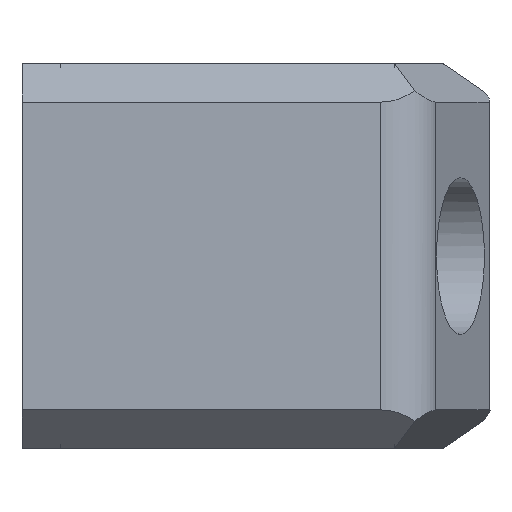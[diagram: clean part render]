
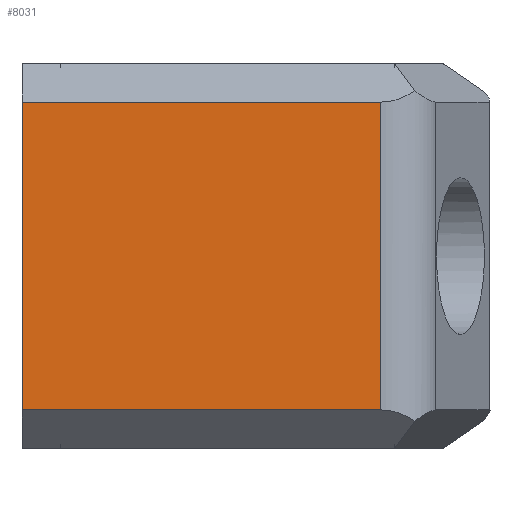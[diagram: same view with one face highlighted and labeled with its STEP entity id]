
A CAD part, left-side view. The second image highlights one B-rep face of the part: STEP entity #8031.
In plain terms, the highlighted planar face has unit normal (-1, 0, 0).
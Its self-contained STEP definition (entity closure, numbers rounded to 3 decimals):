
#233=PLANE('',#8473);
#665=FACE_OUTER_BOUND('',#1100,.T.);
#1100=EDGE_LOOP('',(#5845,#5846,#5847,#5848));
#1524=LINE('',#10746,#2566);
#1534=LINE('',#12873,#2576);
#1538=LINE('',#12881,#2580);
#1539=LINE('',#12882,#2581);
#2566=VECTOR('',#8887,10.);
#2576=VECTOR('',#8939,10.);
#2580=VECTOR('',#8945,10.);
#2581=VECTOR('',#8946,10.);
#3623=VERTEX_POINT('',#10743);
#3624=VERTEX_POINT('',#10745);
#3702=VERTEX_POINT('',#12872);
#3705=VERTEX_POINT('',#12880);
#4420=EDGE_CURVE('',#3623,#3624,#1524,.T.);
#4535=EDGE_CURVE('',#3624,#3702,#1534,.T.);
#4539=EDGE_CURVE('',#3705,#3623,#1538,.T.);
#4540=EDGE_CURVE('',#3702,#3705,#1539,.T.);
#5845=ORIENTED_EDGE('',*,*,#4420,.F.);
#5846=ORIENTED_EDGE('',*,*,#4539,.F.);
#5847=ORIENTED_EDGE('',*,*,#4540,.F.);
#5848=ORIENTED_EDGE('',*,*,#4535,.F.);
#8031=ADVANCED_FACE('',(#665),#233,.T.);
#8473=AXIS2_PLACEMENT_3D('',#12879,#8943,#8944);
#8887=DIRECTION('',(0.,0.,-1.));
#8939=DIRECTION('',(0.,1.,0.));
#8943=DIRECTION('center_axis',(-1.,0.,0.));
#8944=DIRECTION('ref_axis',(0.,1.,0.));
#8945=DIRECTION('',(0.,-1.,0.));
#8946=DIRECTION('',(0.,0.,1.));
#10743=CARTESIAN_POINT('',(331.582,85.339,172.996));
#10745=CARTESIAN_POINT('',(331.582,85.339,156.996));
#10746=CARTESIAN_POINT('',(331.582,85.339,164.996));
#12872=CARTESIAN_POINT('',(331.582,103.957,156.996));
#12873=CARTESIAN_POINT('',(331.582,87.325,156.996));
#12879=CARTESIAN_POINT('Origin',(331.582,83.117,164.996));
#12880=CARTESIAN_POINT('',(331.582,103.957,172.996));
#12881=CARTESIAN_POINT('',(331.582,87.325,172.996));
#12882=CARTESIAN_POINT('',(331.582,103.957,164.996));
